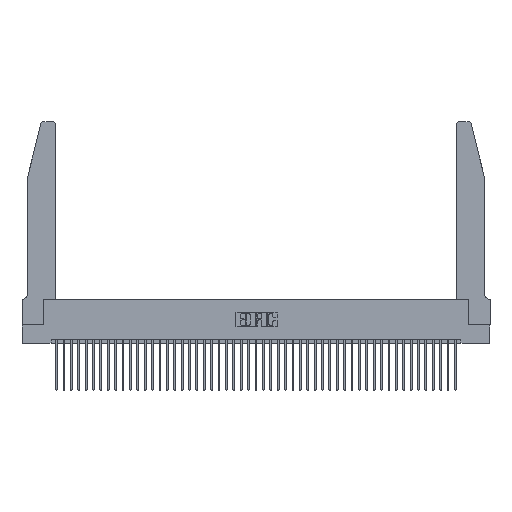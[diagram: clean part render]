
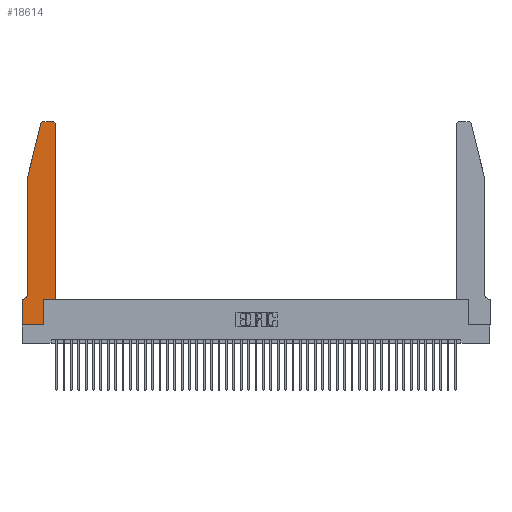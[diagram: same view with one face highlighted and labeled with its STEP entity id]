
A CAD part, top view. The second image highlights one B-rep face of the part: STEP entity #18614.
In plain terms, the highlighted planar face has unit normal (0, 0, 1).
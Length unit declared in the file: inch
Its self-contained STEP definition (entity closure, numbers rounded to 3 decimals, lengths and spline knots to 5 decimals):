
#583 = AXIS2_PLACEMENT_3D ( 'NONE', #28796, #7454, #32357 ) ;
#1818 = ORIENTED_EDGE ( 'NONE', *, *, #11932, .T. ) ;
#2058 = CARTESIAN_POINT ( 'NONE',  ( 0.0755, 2., 0.37 ) ) ;
#3927 = ORIENTED_EDGE ( 'NONE', *, *, #15657, .T. ) ;
#4017 = EDGE_CURVE ( 'NONE', #33670, #15813, #35450, .T. ) ;
#4481 = ORIENTED_EDGE ( 'NONE', *, *, #34239, .T. ) ;
#4660 = VERTEX_POINT ( 'NONE', #37777 ) ;
#6518 = VECTOR ( 'NONE', #22317, 39.37008 ) ;
#6736 = EDGE_CURVE ( 'NONE', #27486, #19350, #9799, .T. ) ;
#7454 = DIRECTION ( 'NONE',  ( 0., 0., 1. ) ) ;
#7629 = EDGE_CURVE ( 'NONE', #43144, #39190, #31812, .T. ) ;
#7700 = EDGE_CURVE ( 'NONE', #39190, #27486, #37937, .T. ) ;
#8458 = CARTESIAN_POINT ( 'NONE',  ( 0.4205, 2.72, 0.37 ) ) ;
#8536 = CARTESIAN_POINT ( 'NONE',  ( 0.4505, 2.72, 0.37 ) ) ;
#8675 = EDGE_LOOP ( 'NONE', ( #29232, #31352, #37991, #4481, #23431, #1818, #25603, #3927, #32326, #23064, #16335, #37021 ) ) ;
#8980 = CARTESIAN_POINT ( 'NONE',  ( 0.4205, 2.75, 0.37 ) ) ;
#9377 = EDGE_CURVE ( 'NONE', #39655, #42526, #36746, .T. ) ;
#9799 = CIRCLE ( 'NONE', #28805, 0.03 ) ;
#9987 = CARTESIAN_POINT ( 'NONE',  ( 0.4505, 0.35, 0.37 ) ) ;
#10765 = CARTESIAN_POINT ( 'NONE',  ( 0.4505, 0.35, 0.37 ) ) ;
#11548 = DIRECTION ( 'NONE',  ( 0., 0., 1. ) ) ;
#11932 = EDGE_CURVE ( 'NONE', #42526, #14509, #39794, .T. ) ;
#12072 = DIRECTION ( 'NONE',  ( 1., 0., 0. ) ) ;
#12255 = CARTESIAN_POINT ( 'NONE',  ( 0., 0., 0.37 ) ) ;
#12359 = DIRECTION ( 'NONE',  ( 0., 0., -1. ) ) ;
#13096 = AXIS2_PLACEMENT_3D ( 'NONE', #33640, #12359, #37213 ) ;
#14384 = VECTOR ( 'NONE', #21546, 39.37008 ) ;
#14509 = VERTEX_POINT ( 'NONE', #41015 ) ;
#14795 = CARTESIAN_POINT ( 'NONE',  ( 0., 0.35, 0.37 ) ) ;
#15107 = EDGE_CURVE ( 'NONE', #14509, #4660, #30001, .T. ) ;
#15145 = DIRECTION ( 'NONE',  ( -1., 0., 0. ) ) ;
#15657 = EDGE_CURVE ( 'NONE', #4660, #19671, #26631, .T. ) ;
#15813 = VERTEX_POINT ( 'NONE', #44930 ) ;
#16335 = ORIENTED_EDGE ( 'NONE', *, *, #7700, .T. ) ;
#17471 = LINE ( 'NONE', #22148, #43590 ) ;
#17960 = CARTESIAN_POINT ( 'NONE',  ( 0.0755, 2., 0.37 ) ) ;
#18614 = ADVANCED_FACE ( 'NONE', ( #30018 ), #35929, .T. ) ;
#18721 = CARTESIAN_POINT ( 'NONE',  ( 0., 0., 0.37 ) ) ;
#18904 = VECTOR ( 'NONE', #45103, 39.37008 ) ;
#19350 = VERTEX_POINT ( 'NONE', #8980 ) ;
#19671 = VERTEX_POINT ( 'NONE', #28380 ) ;
#20577 = VECTOR ( 'NONE', #40658, 39.37008 ) ;
#21546 = DIRECTION ( 'NONE',  ( 0., -1., 0. ) ) ;
#22148 = CARTESIAN_POINT ( 'NONE',  ( 0.2605, 2.75, 0.37 ) ) ;
#22317 = DIRECTION ( 'NONE',  ( 1., 0., 0. ) ) ;
#22382 = CARTESIAN_POINT ( 'NONE',  ( 0.284, 2.75, 0.37 ) ) ;
#22813 = EDGE_CURVE ( 'NONE', #19350, #43333, #17471, .T. ) ;
#23064 = ORIENTED_EDGE ( 'NONE', *, *, #7629, .T. ) ;
#23431 = ORIENTED_EDGE ( 'NONE', *, *, #9377, .T. ) ;
#25157 = CARTESIAN_POINT ( 'NONE',  ( 0.0755, 0.42, 0.37 ) ) ;
#25603 = ORIENTED_EDGE ( 'NONE', *, *, #15107, .T. ) ;
#25652 = CARTESIAN_POINT ( 'NONE',  ( 0.4505, 0.35, 0.37 ) ) ;
#26631 = LINE ( 'NONE', #18721, #6518 ) ;
#27086 = VECTOR ( 'NONE', #30654, 39.37008 ) ;
#27164 = LINE ( 'NONE', #17960, #14384 ) ;
#27486 = VERTEX_POINT ( 'NONE', #8536 ) ;
#27837 = DIRECTION ( 'NONE',  ( 1., 0., 0. ) ) ;
#28380 = CARTESIAN_POINT ( 'NONE',  ( 0.2865, 0., 0.37 ) ) ;
#28497 = CARTESIAN_POINT ( 'NONE',  ( 0.2865, 0.35, 0.37 ) ) ;
#28713 = CARTESIAN_POINT ( 'NONE',  ( 0.0755, 0.35, 0.37 ) ) ;
#28796 = CARTESIAN_POINT ( 'NONE',  ( 0.284, 2.72, 0.37 ) ) ;
#28805 = AXIS2_PLACEMENT_3D ( 'NONE', #8458, #33339, #12072 ) ;
#29218 = VECTOR ( 'NONE', #32127, 39.37008 ) ;
#29232 = ORIENTED_EDGE ( 'NONE', *, *, #22813, .T. ) ;
#29464 = LINE ( 'NONE', #41558, #18904 ) ;
#29581 = VECTOR ( 'NONE', #39178, 39.37008 ) ;
#30001 = LINE ( 'NONE', #12255, #20577 ) ;
#30018 = FACE_OUTER_BOUND ( 'NONE', #8675, .T. ) ;
#30654 = DIRECTION ( 'NONE',  ( -0.239, -0.971, 0. ) ) ;
#30687 = VECTOR ( 'NONE', #27837, 39.37008 ) ;
#31352 = ORIENTED_EDGE ( 'NONE', *, *, #46021, .T. ) ;
#31812 = LINE ( 'NONE', #9987, #30687 ) ;
#32127 = DIRECTION ( 'NONE',  ( -1., 0., 0. ) ) ;
#32326 = ORIENTED_EDGE ( 'NONE', *, *, #45760, .T. ) ;
#32357 = DIRECTION ( 'NONE',  ( 1., 0., 0. ) ) ;
#33339 = DIRECTION ( 'NONE',  ( 0., 0., 1. ) ) ;
#33640 = CARTESIAN_POINT ( 'NONE',  ( 0.0055, 0.42, 0.37 ) ) ;
#33670 = VERTEX_POINT ( 'NONE', #36197 ) ;
#34239 = EDGE_CURVE ( 'NONE', #15813, #39655, #27164, .T. ) ;
#34434 = CIRCLE ( 'NONE', #583, 0.03 ) ;
#35450 = LINE ( 'NONE', #2058, #27086 ) ;
#35929 = PLANE ( 'NONE',  #35975 ) ;
#35975 = AXIS2_PLACEMENT_3D ( 'NONE', #14795, #11548, #36402 ) ;
#36197 = CARTESIAN_POINT ( 'NONE',  ( 0.25487, 2.72718, 0.37 ) ) ;
#36402 = DIRECTION ( 'NONE',  ( 1., 0., 0. ) ) ;
#36746 = CIRCLE ( 'NONE', #13096, 0.07 ) ;
#37021 = ORIENTED_EDGE ( 'NONE', *, *, #6736, .T. ) ;
#37213 = DIRECTION ( 'NONE',  ( -1., 0., 0. ) ) ;
#37777 = CARTESIAN_POINT ( 'NONE',  ( 0., 0., 0.37 ) ) ;
#37937 = LINE ( 'NONE', #10765, #29581 ) ;
#37991 = ORIENTED_EDGE ( 'NONE', *, *, #4017, .T. ) ;
#39178 = DIRECTION ( 'NONE',  ( 0., 1., 0. ) ) ;
#39190 = VERTEX_POINT ( 'NONE', #25652 ) ;
#39655 = VERTEX_POINT ( 'NONE', #25157 ) ;
#39794 = LINE ( 'NONE', #28713, #29218 ) ;
#40658 = DIRECTION ( 'NONE',  ( 0., -1., 0. ) ) ;
#41015 = CARTESIAN_POINT ( 'NONE',  ( 0., 0.35, 0.37 ) ) ;
#41558 = CARTESIAN_POINT ( 'NONE',  ( 0.2865, 0.35, 0.37 ) ) ;
#42131 = CARTESIAN_POINT ( 'NONE',  ( 0.0055, 0.35, 0.37 ) ) ;
#42526 = VERTEX_POINT ( 'NONE', #42131 ) ;
#43144 = VERTEX_POINT ( 'NONE', #28497 ) ;
#43333 = VERTEX_POINT ( 'NONE', #22382 ) ;
#43590 = VECTOR ( 'NONE', #15145, 39.37008 ) ;
#44930 = CARTESIAN_POINT ( 'NONE',  ( 0.0755, 2., 0.37 ) ) ;
#45103 = DIRECTION ( 'NONE',  ( 0., 1., 0. ) ) ;
#45760 = EDGE_CURVE ( 'NONE', #19671, #43144, #29464, .T. ) ;
#46021 = EDGE_CURVE ( 'NONE', #43333, #33670, #34434, .T. ) ;
